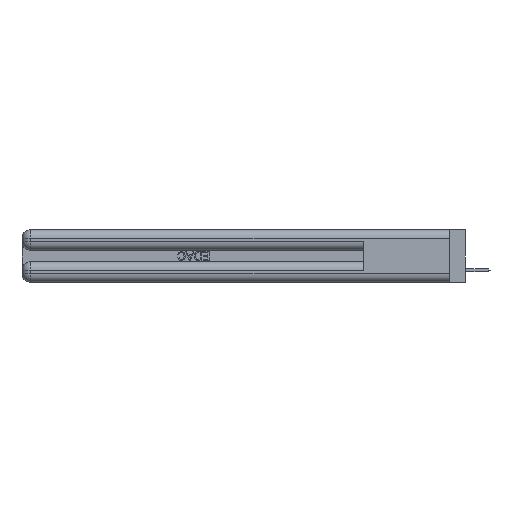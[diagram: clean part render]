
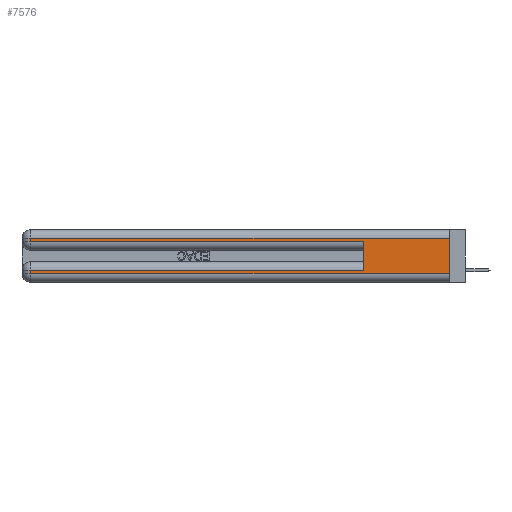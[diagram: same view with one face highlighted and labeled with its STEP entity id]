
A CAD part, left-side view. The second image highlights one B-rep face of the part: STEP entity #7576.
In plain terms, the highlighted planar face has unit normal (-1, 0, 0).
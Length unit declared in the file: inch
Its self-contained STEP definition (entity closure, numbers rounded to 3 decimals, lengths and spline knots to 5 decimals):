
#593 = EDGE_CURVE ( 'NONE', #18073, #39817, #22797, .T. ) ;
#1384 = VECTOR ( 'NONE', #26986, 39.37008 ) ;
#1695 = CARTESIAN_POINT ( 'NONE',  ( 0., 0., 0.06 ) ) ;
#2737 = CARTESIAN_POINT ( 'NONE',  ( 0., 0., 0.31 ) ) ;
#2874 = CARTESIAN_POINT ( 'NONE',  ( 0., 0., 0.37 ) ) ;
#2979 = VERTEX_POINT ( 'NONE', #13533 ) ;
#4231 = EDGE_CURVE ( 'NONE', #2979, #55564, #15008, .T. ) ;
#6085 = DIRECTION ( 'NONE',  ( 0., 0., -1. ) ) ;
#6999 = VECTOR ( 'NONE', #6085, 39.37008 ) ;
#7205 = DIRECTION ( 'NONE',  ( 1., 0., 0. ) ) ;
#7576 = ADVANCED_FACE ( 'NONE', ( #11841 ), #28610, .F. ) ;
#9622 = CARTESIAN_POINT ( 'NONE',  ( 0., 0., 0.085 ) ) ;
#10548 = ORIENTED_EDGE ( 'NONE', *, *, #26818, .T. ) ;
#11055 = ORIENTED_EDGE ( 'NONE', *, *, #4231, .T. ) ;
#11191 = CARTESIAN_POINT ( 'NONE',  ( 0., 0., 0.06 ) ) ;
#11274 = ORIENTED_EDGE ( 'NONE', *, *, #24183, .F. ) ;
#11419 = VECTOR ( 'NONE', #36438, 39.37008 ) ;
#11841 = FACE_OUTER_BOUND ( 'NONE', #52737, .T. ) ;
#11849 = CARTESIAN_POINT ( 'NONE',  ( 0., 2.94, 0.37 ) ) ;
#12307 = LINE ( 'NONE', #1695, #29139 ) ;
#12584 = VERTEX_POINT ( 'NONE', #20147 ) ;
#12991 = VERTEX_POINT ( 'NONE', #35226 ) ;
#13533 = CARTESIAN_POINT ( 'NONE',  ( 0., 0., 0.31 ) ) ;
#15008 = LINE ( 'NONE', #2737, #27033 ) ;
#15122 = CARTESIAN_POINT ( 'NONE',  ( 0., 2.94, 0.31 ) ) ;
#18073 = VERTEX_POINT ( 'NONE', #47016 ) ;
#18537 = EDGE_CURVE ( 'NONE', #18073, #12991, #37550, .T. ) ;
#19907 = VECTOR ( 'NONE', #32867, 39.37008 ) ;
#20147 = CARTESIAN_POINT ( 'NONE',  ( 0., 2.94, 0.285 ) ) ;
#20221 = DIRECTION ( 'NONE',  ( 0., 0., -1. ) ) ;
#20416 = LINE ( 'NONE', #36312, #44476 ) ;
#22217 = CARTESIAN_POINT ( 'NONE',  ( 0., 2.94, 0.085 ) ) ;
#22797 = LINE ( 'NONE', #9622, #11419 ) ;
#22951 = LINE ( 'NONE', #25600, #1384 ) ;
#24183 = EDGE_CURVE ( 'NONE', #2979, #26185, #20416, .T. ) ;
#25600 = CARTESIAN_POINT ( 'NONE',  ( 0., 0., 0.285 ) ) ;
#26185 = VERTEX_POINT ( 'NONE', #11191 ) ;
#26818 = EDGE_CURVE ( 'NONE', #28423, #26185, #12307, .T. ) ;
#26986 = DIRECTION ( 'NONE',  ( 0., -1., 0. ) ) ;
#27033 = VECTOR ( 'NONE', #50259, 39.37008 ) ;
#28423 = VERTEX_POINT ( 'NONE', #47992 ) ;
#28610 = PLANE ( 'NONE',  #28958 ) ;
#28958 = AXIS2_PLACEMENT_3D ( 'NONE', #2874, #7205, #20221 ) ;
#29139 = VECTOR ( 'NONE', #49785, 39.37008 ) ;
#30120 = DIRECTION ( 'NONE',  ( 0., 0., 1. ) ) ;
#30322 = ORIENTED_EDGE ( 'NONE', *, *, #593, .T. ) ;
#30510 = ORIENTED_EDGE ( 'NONE', *, *, #18537, .F. ) ;
#31056 = EDGE_CURVE ( 'NONE', #55564, #12584, #54090, .T. ) ;
#31897 = ORIENTED_EDGE ( 'NONE', *, *, #45781, .T. ) ;
#32867 = DIRECTION ( 'NONE',  ( 0., 0., -1. ) ) ;
#33573 = ORIENTED_EDGE ( 'NONE', *, *, #31056, .T. ) ;
#35226 = CARTESIAN_POINT ( 'NONE',  ( 0., 0.6, 0.285 ) ) ;
#36312 = CARTESIAN_POINT ( 'NONE',  ( 0., 0., 0.37 ) ) ;
#36438 = DIRECTION ( 'NONE',  ( 0., 1., 0. ) ) ;
#36551 = LINE ( 'NONE', #48286, #6999 ) ;
#37550 = LINE ( 'NONE', #43065, #44209 ) ;
#39338 = EDGE_CURVE ( 'NONE', #12584, #12991, #22951, .T. ) ;
#39817 = VERTEX_POINT ( 'NONE', #22217 ) ;
#43065 = CARTESIAN_POINT ( 'NONE',  ( 0., 0.6, 0.145 ) ) ;
#44209 = VECTOR ( 'NONE', #30120, 39.37008 ) ;
#44476 = VECTOR ( 'NONE', #45144, 39.37008 ) ;
#45144 = DIRECTION ( 'NONE',  ( 0., 0., -1. ) ) ;
#45781 = EDGE_CURVE ( 'NONE', #39817, #28423, #36551, .T. ) ;
#47016 = CARTESIAN_POINT ( 'NONE',  ( 0., 0.6, 0.085 ) ) ;
#47992 = CARTESIAN_POINT ( 'NONE',  ( 0., 2.94, 0.06 ) ) ;
#48269 = ORIENTED_EDGE ( 'NONE', *, *, #39338, .T. ) ;
#48286 = CARTESIAN_POINT ( 'NONE',  ( 0., 2.94, 0.37 ) ) ;
#49785 = DIRECTION ( 'NONE',  ( 0., -1., 0. ) ) ;
#50259 = DIRECTION ( 'NONE',  ( 0., 1., 0. ) ) ;
#52737 = EDGE_LOOP ( 'NONE', ( #11274, #11055, #33573, #48269, #30510, #30322, #31897, #10548 ) ) ;
#54090 = LINE ( 'NONE', #11849, #19907 ) ;
#55564 = VERTEX_POINT ( 'NONE', #15122 ) ;
